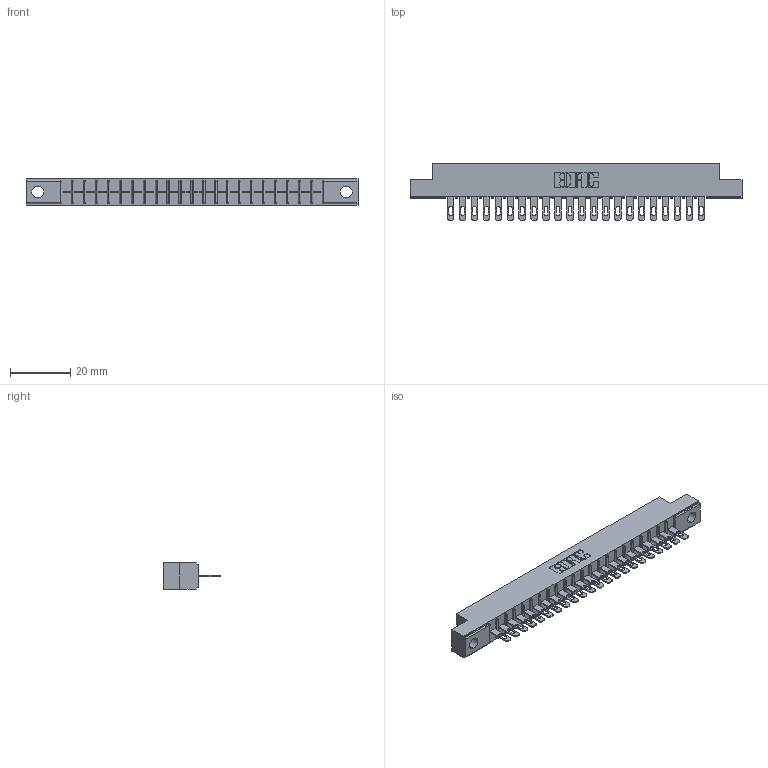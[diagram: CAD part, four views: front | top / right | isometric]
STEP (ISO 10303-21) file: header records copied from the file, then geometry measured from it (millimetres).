
FILE_DESCRIPTION (( 'STEP AP203' ), '1' );
FILE_NAME ('356-022-400-104.STEP', '2020-09-23T15:12:35', ( '' ), ( '' ), 'SwSTEP 2.0', 'SolidWorks 2020', '' );
FILE_SCHEMA (( 'CONFIG_CONTROL_DESIGN' ));
Length unit declared in the file: inch
Products named in the file (3): 356-022-400-104; 306 Part_.156 Dia; 306-290-001_100
Assembly tree (23 placements, depth 2):
  356-022-400-104
    306 Part_.156 Dia
    306-290-001_100  x22
Bounding box: 110.19 x 18.87 x 8.71 mm (x, y, z)
Volume: 7496.6 mm3; surface area: 11306.1 mm2
Topology: 23 solids, 23 shells, 1802 faces, 5082 edges, 3268 vertices
Faces by surface type: plane 1182, cylinder 532, sphere 88
Entity records: 23689 total; most frequent: CARTESIAN_POINT 3979, ORIENTED_EDGE 3940, DIRECTION 3918, EDGE_CURVE 1970, VECTOR 1536, LINE 1536, VERTEX_POINT 1252, AXIS2_PLACEMENT_3D 1191
